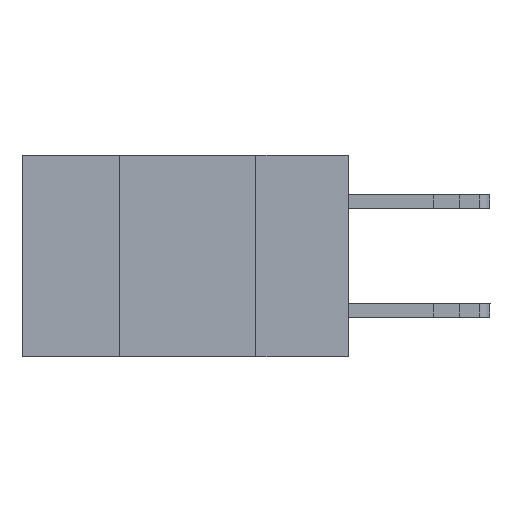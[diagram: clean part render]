
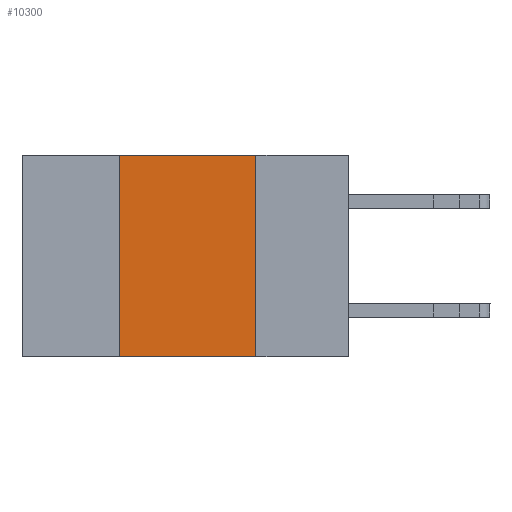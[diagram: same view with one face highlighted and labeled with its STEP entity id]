
A CAD part, left-side view. The second image highlights one B-rep face of the part: STEP entity #10300.
In plain terms, the highlighted planar face has unit normal (-1, 0, 0).
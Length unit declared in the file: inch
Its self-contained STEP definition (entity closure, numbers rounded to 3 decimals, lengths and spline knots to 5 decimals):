
#1106 = CARTESIAN_POINT ( 'NONE',  ( 0., 0.42, 0. ) ) ;
#1218 = ORIENTED_EDGE ( 'NONE', *, *, #12744, .F. ) ;
#1884 = VECTOR ( 'NONE', #11489, 39.37008 ) ;
#2365 = ORIENTED_EDGE ( 'NONE', *, *, #10806, .F. ) ;
#3274 = PLANE ( 'NONE',  #10171 ) ;
#3383 = FACE_OUTER_BOUND ( 'NONE', #5561, .T. ) ;
#3551 = CARTESIAN_POINT ( 'NONE',  ( 0., 0.17, -0.37 ) ) ;
#3772 = CARTESIAN_POINT ( 'NONE',  ( 0., 0.42, -0.37 ) ) ;
#4251 = CARTESIAN_POINT ( 'NONE',  ( 0., 0.6, 0. ) ) ;
#4547 = VERTEX_POINT ( 'NONE', #5955 ) ;
#5222 = LINE ( 'NONE', #4251, #1884 ) ;
#5561 = EDGE_LOOP ( 'NONE', ( #5585, #2365, #1218, #6597 ) ) ;
#5585 = ORIENTED_EDGE ( 'NONE', *, *, #9797, .F. ) ;
#5827 = CARTESIAN_POINT ( 'NONE',  ( 0., 0.6, 0. ) ) ;
#5955 = CARTESIAN_POINT ( 'NONE',  ( 0., 0.17, 0. ) ) ;
#6556 = VECTOR ( 'NONE', #15044, 39.37008 ) ;
#6597 = ORIENTED_EDGE ( 'NONE', *, *, #11964, .T. ) ;
#6722 = VECTOR ( 'NONE', #9430, 39.37008 ) ;
#6924 = LINE ( 'NONE', #6943, #6556 ) ;
#6943 = CARTESIAN_POINT ( 'NONE',  ( 0., 0.6, -0.37 ) ) ;
#7038 = DIRECTION ( 'NONE',  ( 0., 0., -1. ) ) ;
#7294 = DIRECTION ( 'NONE',  ( 0., 0., -1. ) ) ;
#7828 = CARTESIAN_POINT ( 'NONE',  ( 0., 0.17, -0.37 ) ) ;
#8343 = VERTEX_POINT ( 'NONE', #7828 ) ;
#9430 = DIRECTION ( 'NONE',  ( 0., 0., 1. ) ) ;
#9797 = EDGE_CURVE ( 'NONE', #4547, #8343, #10643, .T. ) ;
#10171 = AXIS2_PLACEMENT_3D ( 'NONE', #5827, #14019, #7038 ) ;
#10265 = VECTOR ( 'NONE', #7294, 39.37008 ) ;
#10300 = ADVANCED_FACE ( 'NONE', ( #3383 ), #3274, .F. ) ;
#10622 = CARTESIAN_POINT ( 'NONE',  ( 0., 0.42, -0.37 ) ) ;
#10643 = LINE ( 'NONE', #3551, #10265 ) ;
#10806 = EDGE_CURVE ( 'NONE', #11116, #4547, #5222, .T. ) ;
#11116 = VERTEX_POINT ( 'NONE', #1106 ) ;
#11489 = DIRECTION ( 'NONE',  ( 0., -1., 0. ) ) ;
#11964 = EDGE_CURVE ( 'NONE', #12320, #8343, #6924, .T. ) ;
#12320 = VERTEX_POINT ( 'NONE', #3772 ) ;
#12744 = EDGE_CURVE ( 'NONE', #12320, #11116, #13344, .T. ) ;
#13344 = LINE ( 'NONE', #10622, #6722 ) ;
#14019 = DIRECTION ( 'NONE',  ( 1., 0., 0. ) ) ;
#15044 = DIRECTION ( 'NONE',  ( 0., -1., 0. ) ) ;
